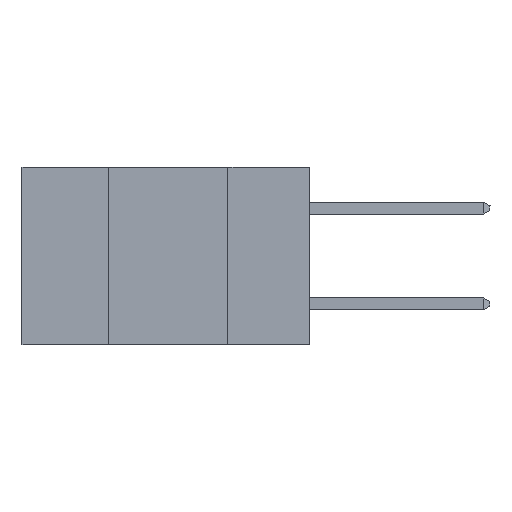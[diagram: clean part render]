
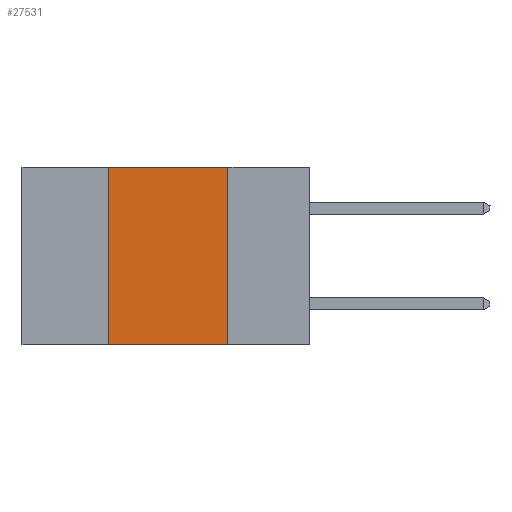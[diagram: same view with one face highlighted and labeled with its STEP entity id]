
A CAD part, left-side view. The second image highlights one B-rep face of the part: STEP entity #27531.
In plain terms, the highlighted planar face has unit normal (-1, 0, 0).
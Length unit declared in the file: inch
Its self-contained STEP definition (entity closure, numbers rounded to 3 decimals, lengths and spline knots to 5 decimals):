
#241 = VECTOR ( 'NONE', #20069, 39.37008 ) ;
#1211 = DIRECTION ( 'NONE',  ( 0., 0., -1. ) ) ;
#1333 = EDGE_LOOP ( 'NONE', ( #26136, #2306, #20063, #18983 ) ) ;
#1345 = CARTESIAN_POINT ( 'NONE',  ( 0., 0.6, 0. ) ) ;
#2306 = ORIENTED_EDGE ( 'NONE', *, *, #28336, .F. ) ;
#2568 = CARTESIAN_POINT ( 'NONE',  ( 0., 0.17, -0.37 ) ) ;
#3237 = AXIS2_PLACEMENT_3D ( 'NONE', #1345, #21612, #1211 ) ;
#3443 = CARTESIAN_POINT ( 'NONE',  ( 0., 0.6, 0. ) ) ;
#5748 = FACE_OUTER_BOUND ( 'NONE', #1333, .T. ) ;
#7250 = VECTOR ( 'NONE', #25594, 39.37008 ) ;
#8150 = LINE ( 'NONE', #3443, #20080 ) ;
#8748 = CARTESIAN_POINT ( 'NONE',  ( 0., 0.17, 0. ) ) ;
#9088 = CARTESIAN_POINT ( 'NONE',  ( 0., 0.6, -0.37 ) ) ;
#9102 = VERTEX_POINT ( 'NONE', #21327 ) ;
#9236 = LINE ( 'NONE', #9088, #21906 ) ;
#12337 = PLANE ( 'NONE',  #3237 ) ;
#13988 = CARTESIAN_POINT ( 'NONE',  ( 0., 0.42, 0. ) ) ;
#15454 = VERTEX_POINT ( 'NONE', #2568 ) ;
#18187 = DIRECTION ( 'NONE',  ( 0., -1., 0. ) ) ;
#18983 = ORIENTED_EDGE ( 'NONE', *, *, #19828, .T. ) ;
#19003 = DIRECTION ( 'NONE',  ( 0., -1., 0. ) ) ;
#19828 = EDGE_CURVE ( 'NONE', #9102, #15454, #9236, .T. ) ;
#20063 = ORIENTED_EDGE ( 'NONE', *, *, #20723, .F. ) ;
#20069 = DIRECTION ( 'NONE',  ( 0., 0., -1. ) ) ;
#20080 = VECTOR ( 'NONE', #19003, 39.37008 ) ;
#20723 = EDGE_CURVE ( 'NONE', #9102, #26281, #23119, .T. ) ;
#21327 = CARTESIAN_POINT ( 'NONE',  ( 0., 0.42, -0.37 ) ) ;
#21329 = EDGE_CURVE ( 'NONE', #27126, #15454, #26249, .T. ) ;
#21612 = DIRECTION ( 'NONE',  ( 1., 0., 0. ) ) ;
#21906 = VECTOR ( 'NONE', #18187, 39.37008 ) ;
#23119 = LINE ( 'NONE', #13988, #7250 ) ;
#25594 = DIRECTION ( 'NONE',  ( 0., 0., 1. ) ) ;
#26136 = ORIENTED_EDGE ( 'NONE', *, *, #21329, .F. ) ;
#26249 = LINE ( 'NONE', #26391, #241 ) ;
#26281 = VERTEX_POINT ( 'NONE', #27883 ) ;
#26391 = CARTESIAN_POINT ( 'NONE',  ( 0., 0.17, 0. ) ) ;
#27126 = VERTEX_POINT ( 'NONE', #8748 ) ;
#27531 = ADVANCED_FACE ( 'NONE', ( #5748 ), #12337, .F. ) ;
#27883 = CARTESIAN_POINT ( 'NONE',  ( 0., 0.42, 0. ) ) ;
#28336 = EDGE_CURVE ( 'NONE', #26281, #27126, #8150, .T. ) ;
